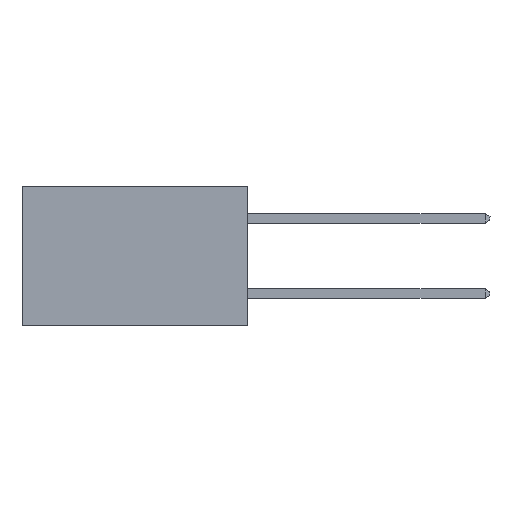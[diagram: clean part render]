
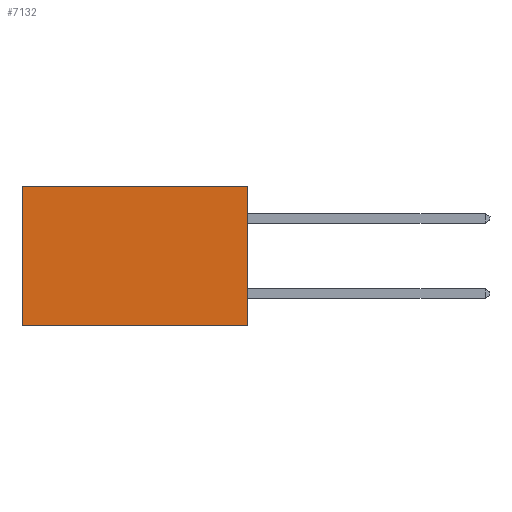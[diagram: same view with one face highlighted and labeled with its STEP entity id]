
A CAD part, left-side view. The second image highlights one B-rep face of the part: STEP entity #7132.
In plain terms, the highlighted planar face has unit normal (-1, 0, 0).
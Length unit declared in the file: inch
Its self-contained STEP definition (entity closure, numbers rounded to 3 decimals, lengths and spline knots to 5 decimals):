
#824 = VECTOR ( 'NONE', #10308, 39.37008 ) ;
#1182 = EDGE_CURVE ( 'NONE', #8210, #7524, #6534, .T. ) ;
#1917 = VERTEX_POINT ( 'NONE', #8321 ) ;
#2242 = ORIENTED_EDGE ( 'NONE', *, *, #7214, .F. ) ;
#2567 = CARTESIAN_POINT ( 'NONE',  ( 0.298, 0., 0. ) ) ;
#3433 = CARTESIAN_POINT ( 'NONE',  ( 0.298, 0., 0. ) ) ;
#3636 = FACE_OUTER_BOUND ( 'NONE', #6406, .T. ) ;
#3732 = LINE ( 'NONE', #2567, #824 ) ;
#4301 = VECTOR ( 'NONE', #8279, 39.37008 ) ;
#4496 = PLANE ( 'NONE',  #7313 ) ;
#5145 = CARTESIAN_POINT ( 'NONE',  ( 0.298, 0.6, 0. ) ) ;
#5532 = ORIENTED_EDGE ( 'NONE', *, *, #13573, .T. ) ;
#6406 = EDGE_LOOP ( 'NONE', ( #7859, #2242, #12401, #5532 ) ) ;
#6534 = LINE ( 'NONE', #5145, #13607 ) ;
#7132 = ADVANCED_FACE ( 'NONE', ( #3636 ), #4496, .F. ) ;
#7214 = EDGE_CURVE ( 'NONE', #1917, #7524, #13793, .T. ) ;
#7313 = AXIS2_PLACEMENT_3D ( 'NONE', #3433, #12254, #13240 ) ;
#7371 = DIRECTION ( 'NONE',  ( 0., 0., -1. ) ) ;
#7524 = VERTEX_POINT ( 'NONE', #8009 ) ;
#7859 = ORIENTED_EDGE ( 'NONE', *, *, #1182, .T. ) ;
#8009 = CARTESIAN_POINT ( 'NONE',  ( 0.298, 0.6, -0.37 ) ) ;
#8014 = LINE ( 'NONE', #12934, #11782 ) ;
#8210 = VERTEX_POINT ( 'NONE', #14198 ) ;
#8279 = DIRECTION ( 'NONE',  ( 0., 1., 0. ) ) ;
#8321 = CARTESIAN_POINT ( 'NONE',  ( 0.298, 0., -0.37 ) ) ;
#9409 = EDGE_CURVE ( 'NONE', #12653, #1917, #3732, .T. ) ;
#9611 = DIRECTION ( 'NONE',  ( 0., 1., 0. ) ) ;
#10308 = DIRECTION ( 'NONE',  ( 0., 0., -1. ) ) ;
#11672 = CARTESIAN_POINT ( 'NONE',  ( 0.298, 0., -0.37 ) ) ;
#11782 = VECTOR ( 'NONE', #9611, 39.37008 ) ;
#12081 = CARTESIAN_POINT ( 'NONE',  ( 0.298, 0., 0. ) ) ;
#12254 = DIRECTION ( 'NONE',  ( 1., 0., 0. ) ) ;
#12401 = ORIENTED_EDGE ( 'NONE', *, *, #9409, .F. ) ;
#12653 = VERTEX_POINT ( 'NONE', #12081 ) ;
#12934 = CARTESIAN_POINT ( 'NONE',  ( 0.298, 0., 0. ) ) ;
#13240 = DIRECTION ( 'NONE',  ( 0., 0., -1. ) ) ;
#13573 = EDGE_CURVE ( 'NONE', #12653, #8210, #8014, .T. ) ;
#13607 = VECTOR ( 'NONE', #7371, 39.37008 ) ;
#13793 = LINE ( 'NONE', #11672, #4301 ) ;
#14198 = CARTESIAN_POINT ( 'NONE',  ( 0.298, 0.6, 0. ) ) ;
